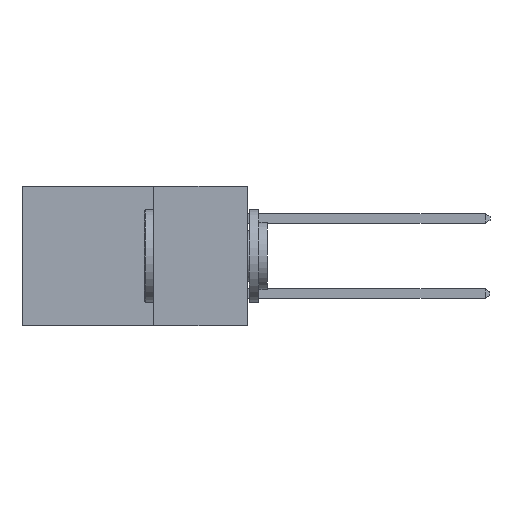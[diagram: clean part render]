
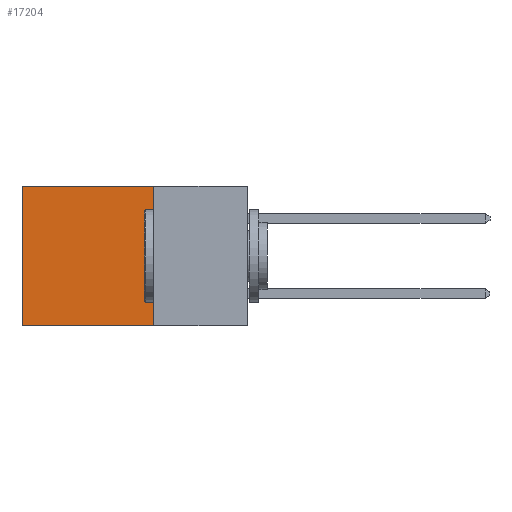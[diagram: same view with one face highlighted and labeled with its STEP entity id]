
A CAD part, left-side view. The second image highlights one B-rep face of the part: STEP entity #17204.
In plain terms, the highlighted planar face has unit normal (-1, 0, 0).
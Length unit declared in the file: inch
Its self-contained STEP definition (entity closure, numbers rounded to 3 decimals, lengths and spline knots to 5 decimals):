
#433 = LINE ( 'NONE', #20759, #1607 ) ;
#611 = EDGE_LOOP ( 'NONE', ( #19866, #18809, #3078, #13728 ) ) ;
#1086 = VECTOR ( 'NONE', #20735, 39.37008 ) ;
#1607 = VECTOR ( 'NONE', #9929, 39.37008 ) ;
#1744 = VERTEX_POINT ( 'NONE', #18601 ) ;
#1998 = PLANE ( 'NONE',  #7973 ) ;
#3078 = ORIENTED_EDGE ( 'NONE', *, *, #20881, .F. ) ;
#4029 = CARTESIAN_POINT ( 'NONE',  ( 0.298, 0.25, -0.37 ) ) ;
#5715 = DIRECTION ( 'NONE',  ( 0., 0., -1. ) ) ;
#6184 = CARTESIAN_POINT ( 'NONE',  ( 0.298, 0.25, 0. ) ) ;
#7973 = AXIS2_PLACEMENT_3D ( 'NONE', #14822, #16677, #5715 ) ;
#9929 = DIRECTION ( 'NONE',  ( 0., 1., 0. ) ) ;
#10925 = LINE ( 'NONE', #6184, #1086 ) ;
#11649 = CARTESIAN_POINT ( 'NONE',  ( 0.298, 0.6, -0.37 ) ) ;
#12428 = VERTEX_POINT ( 'NONE', #16750 ) ;
#12603 = CARTESIAN_POINT ( 'NONE',  ( 0.298, 0.25, -0.37 ) ) ;
#13728 = ORIENTED_EDGE ( 'NONE', *, *, #22212, .T. ) ;
#14137 = EDGE_CURVE ( 'NONE', #23504, #16384, #20994, .T. ) ;
#14615 = DIRECTION ( 'NONE',  ( 0., 0., -1. ) ) ;
#14655 = CARTESIAN_POINT ( 'NONE',  ( 0.298, 0.6, 0. ) ) ;
#14822 = CARTESIAN_POINT ( 'NONE',  ( 0.298, 0.25, 0. ) ) ;
#16192 = VECTOR ( 'NONE', #16258, 39.37008 ) ;
#16258 = DIRECTION ( 'NONE',  ( 0., 1., 0. ) ) ;
#16384 = VERTEX_POINT ( 'NONE', #11649 ) ;
#16677 = DIRECTION ( 'NONE',  ( 1., 0., 0. ) ) ;
#16750 = CARTESIAN_POINT ( 'NONE',  ( 0.298, 0.25, 0. ) ) ;
#16830 = EDGE_CURVE ( 'NONE', #1744, #16384, #20609, .T. ) ;
#17204 = ADVANCED_FACE ( 'NONE', ( #18091 ), #1998, .F. ) ;
#18091 = FACE_OUTER_BOUND ( 'NONE', #611, .T. ) ;
#18601 = CARTESIAN_POINT ( 'NONE',  ( 0.298, 0.6, 0. ) ) ;
#18809 = ORIENTED_EDGE ( 'NONE', *, *, #14137, .F. ) ;
#19866 = ORIENTED_EDGE ( 'NONE', *, *, #16830, .T. ) ;
#20609 = LINE ( 'NONE', #14655, #21178 ) ;
#20735 = DIRECTION ( 'NONE',  ( 0., 0., -1. ) ) ;
#20759 = CARTESIAN_POINT ( 'NONE',  ( 0.298, 0.25, 0. ) ) ;
#20881 = EDGE_CURVE ( 'NONE', #12428, #23504, #10925, .T. ) ;
#20994 = LINE ( 'NONE', #12603, #16192 ) ;
#21178 = VECTOR ( 'NONE', #14615, 39.37008 ) ;
#22212 = EDGE_CURVE ( 'NONE', #12428, #1744, #433, .T. ) ;
#23504 = VERTEX_POINT ( 'NONE', #4029 ) ;
